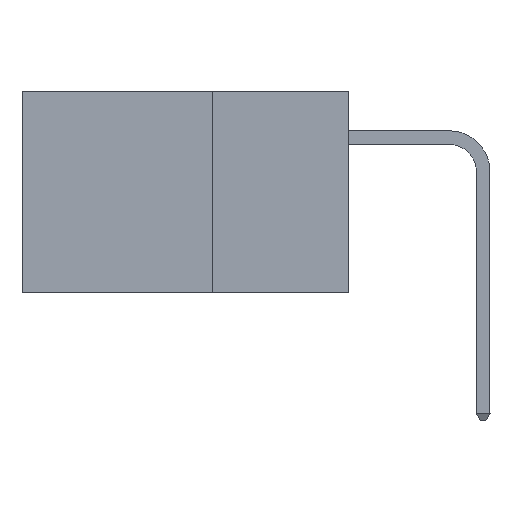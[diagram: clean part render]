
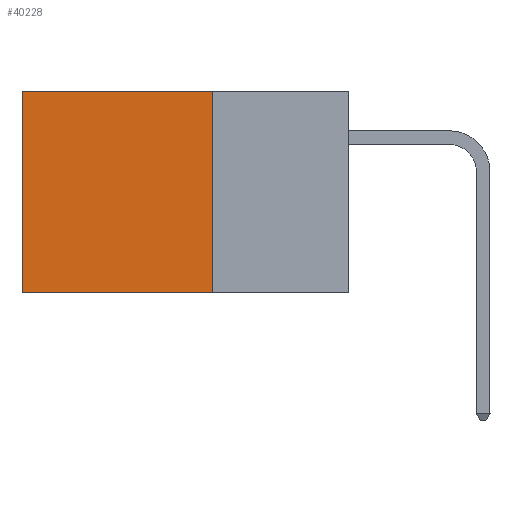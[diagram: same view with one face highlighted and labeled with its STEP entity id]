
A CAD part, left-side view. The second image highlights one B-rep face of the part: STEP entity #40228.
In plain terms, the highlighted planar face has unit normal (-1, 0, 0).
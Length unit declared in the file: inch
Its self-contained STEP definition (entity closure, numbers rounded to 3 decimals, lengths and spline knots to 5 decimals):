
#26 = DIRECTION ( 'NONE',  ( 0., 1., 0. ) ) ;
#316 = DIRECTION ( 'NONE',  ( 0., 0., -1. ) ) ;
#1165 = CARTESIAN_POINT ( 'NONE',  ( 0.2875, 0.25, -0.37 ) ) ;
#2289 = ORIENTED_EDGE ( 'NONE', *, *, #17399, .F. ) ;
#3919 = DIRECTION ( 'NONE',  ( 0., 0., -1. ) ) ;
#4815 = ORIENTED_EDGE ( 'NONE', *, *, #30341, .T. ) ;
#5199 = VERTEX_POINT ( 'NONE', #15992 ) ;
#5341 = CARTESIAN_POINT ( 'NONE',  ( 0.2875, 0.25, 0. ) ) ;
#5774 = DIRECTION ( 'NONE',  ( 0., 1., 0. ) ) ;
#7223 = LINE ( 'NONE', #28994, #20375 ) ;
#8086 = CARTESIAN_POINT ( 'NONE',  ( 0.2875, 0.25, 0. ) ) ;
#10059 = CARTESIAN_POINT ( 'NONE',  ( 0.2875, 0.25, 0. ) ) ;
#10253 = EDGE_LOOP ( 'NONE', ( #34736, #39503, #2289, #4815 ) ) ;
#10865 = EDGE_CURVE ( 'NONE', #34099, #30525, #35117, .T. ) ;
#15199 = LINE ( 'NONE', #8086, #36413 ) ;
#15992 = CARTESIAN_POINT ( 'NONE',  ( 0.2875, 0.25, -0.37 ) ) ;
#17017 = AXIS2_PLACEMENT_3D ( 'NONE', #10059, #22831, #35606 ) ;
#17399 = EDGE_CURVE ( 'NONE', #21442, #5199, #7223, .T. ) ;
#17695 = LINE ( 'NONE', #1165, #35062 ) ;
#20375 = VECTOR ( 'NONE', #316, 39.37008 ) ;
#21442 = VERTEX_POINT ( 'NONE', #5341 ) ;
#22831 = DIRECTION ( 'NONE',  ( 1., 0., 0. ) ) ;
#25022 = VECTOR ( 'NONE', #3919, 39.37008 ) ;
#25978 = FACE_OUTER_BOUND ( 'NONE', #10253, .T. ) ;
#28780 = CARTESIAN_POINT ( 'NONE',  ( 0.2875, 0.6, -0.37 ) ) ;
#28994 = CARTESIAN_POINT ( 'NONE',  ( 0.2875, 0.25, 0. ) ) ;
#30341 = EDGE_CURVE ( 'NONE', #21442, #34099, #15199, .T. ) ;
#30445 = CARTESIAN_POINT ( 'NONE',  ( 0.2875, 0.6, 0. ) ) ;
#30525 = VERTEX_POINT ( 'NONE', #28780 ) ;
#34099 = VERTEX_POINT ( 'NONE', #30445 ) ;
#34736 = ORIENTED_EDGE ( 'NONE', *, *, #10865, .T. ) ;
#35062 = VECTOR ( 'NONE', #26, 39.37008 ) ;
#35117 = LINE ( 'NONE', #35733, #25022 ) ;
#35606 = DIRECTION ( 'NONE',  ( 0., 0., -1. ) ) ;
#35733 = CARTESIAN_POINT ( 'NONE',  ( 0.2875, 0.6, 0. ) ) ;
#36413 = VECTOR ( 'NONE', #5774, 39.37008 ) ;
#38760 = PLANE ( 'NONE',  #17017 ) ;
#39503 = ORIENTED_EDGE ( 'NONE', *, *, #39971, .F. ) ;
#39971 = EDGE_CURVE ( 'NONE', #5199, #30525, #17695, .T. ) ;
#40228 = ADVANCED_FACE ( 'NONE', ( #25978 ), #38760, .F. ) ;
